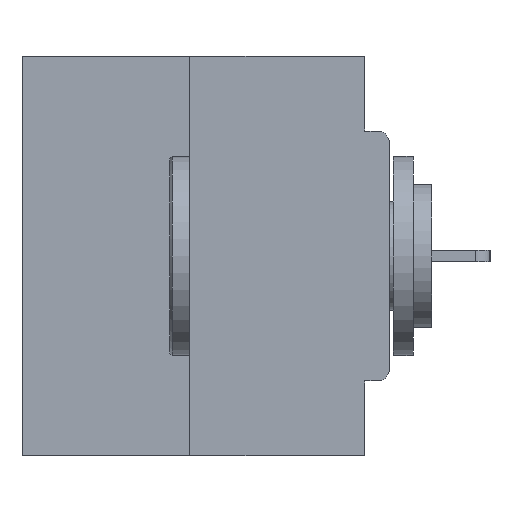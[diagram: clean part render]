
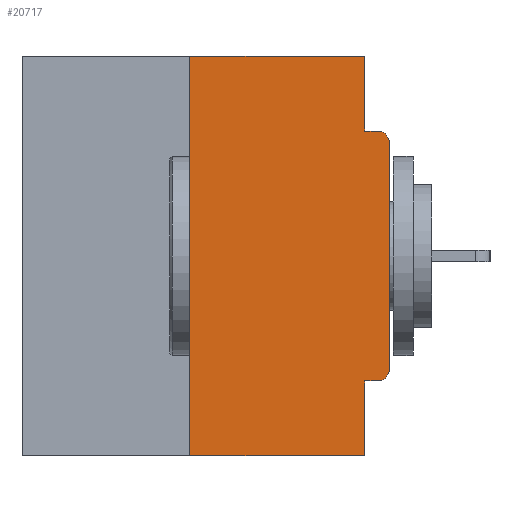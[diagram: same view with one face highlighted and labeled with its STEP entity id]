
A CAD part, left-side view. The second image highlights one B-rep face of the part: STEP entity #20717.
In plain terms, the highlighted planar face has unit normal (-1, 0, 0).
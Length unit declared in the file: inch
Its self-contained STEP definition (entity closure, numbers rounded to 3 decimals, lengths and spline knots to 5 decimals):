
#76 = DIRECTION ( 'NONE',  ( 0., 0., 1. ) ) ;
#214 = VECTOR ( 'NONE', #10319, 39.37008 ) ;
#393 = CARTESIAN_POINT ( 'NONE',  ( 0., 0.46, 0. ) ) ;
#696 = VERTEX_POINT ( 'NONE', #19308 ) ;
#1571 = DIRECTION ( 'NONE',  ( -1., 0., 0. ) ) ;
#2668 = ORIENTED_EDGE ( 'NONE', *, *, #12306, .F. ) ;
#3472 = LINE ( 'NONE', #29844, #12687 ) ;
#3870 = CARTESIAN_POINT ( 'NONE',  ( 0., 0.031, 0. ) ) ;
#4106 = DIRECTION ( 'NONE',  ( 0., 0., -1. ) ) ;
#4189 = PLANE ( 'NONE',  #5320 ) ;
#4296 = DIRECTION ( 'NONE',  ( 0., 0., -1. ) ) ;
#4520 = CARTESIAN_POINT ( 'NONE',  ( 0., 0.015, -0.0935 ) ) ;
#4551 = VERTEX_POINT ( 'NONE', #28477 ) ;
#4788 = VECTOR ( 'NONE', #9952, 39.37008 ) ;
#5167 = VERTEX_POINT ( 'NONE', #29024 ) ;
#5266 = ORIENTED_EDGE ( 'NONE', *, *, #14799, .T. ) ;
#5320 = AXIS2_PLACEMENT_3D ( 'NONE', #6669, #30104, #4296 ) ;
#5883 = EDGE_CURVE ( 'NONE', #19511, #30200, #10725, .T. ) ;
#6249 = VECTOR ( 'NONE', #29331, 39.37008 ) ;
#6626 = ORIENTED_EDGE ( 'NONE', *, *, #5883, .F. ) ;
#6669 = CARTESIAN_POINT ( 'NONE',  ( 0., 0.46, 0. ) ) ;
#6831 = CARTESIAN_POINT ( 'NONE',  ( 0., 0., -0.4065 ) ) ;
#7285 = CARTESIAN_POINT ( 'NONE',  ( 0., 0.031, -0.5 ) ) ;
#8196 = AXIS2_PLACEMENT_3D ( 'NONE', #8327, #22698, #8529 ) ;
#8265 = DIRECTION ( 'NONE',  ( 0., -1., 0. ) ) ;
#8327 = CARTESIAN_POINT ( 'NONE',  ( 0., 0.015, -0.3915 ) ) ;
#8529 = DIRECTION ( 'NONE',  ( 0., 0., -1. ) ) ;
#9159 = VECTOR ( 'NONE', #8265, 39.37008 ) ;
#9408 = CARTESIAN_POINT ( 'NONE',  ( 0., 0.25, 0. ) ) ;
#9952 = DIRECTION ( 'NONE',  ( 0., 0., -1. ) ) ;
#10228 = DIRECTION ( 'NONE',  ( 0., -1., 0. ) ) ;
#10319 = DIRECTION ( 'NONE',  ( 0., 0., 1. ) ) ;
#10347 = CARTESIAN_POINT ( 'NONE',  ( 0., 0.031, -0.4065 ) ) ;
#10432 = CARTESIAN_POINT ( 'NONE',  ( 0., 0., -0.0935 ) ) ;
#10725 = LINE ( 'NONE', #7285, #4788 ) ;
#11297 = VECTOR ( 'NONE', #76, 39.37008 ) ;
#11417 = EDGE_CURVE ( 'NONE', #5167, #19511, #12027, .T. ) ;
#11692 = ORIENTED_EDGE ( 'NONE', *, *, #18692, .T. ) ;
#11786 = ORIENTED_EDGE ( 'NONE', *, *, #16919, .T. ) ;
#12027 = LINE ( 'NONE', #6831, #17896 ) ;
#12306 = EDGE_CURVE ( 'NONE', #4551, #24240, #27589, .T. ) ;
#12375 = CARTESIAN_POINT ( 'NONE',  ( 0., 0., 0. ) ) ;
#12687 = VECTOR ( 'NONE', #15627, 39.37008 ) ;
#12829 = CARTESIAN_POINT ( 'NONE',  ( 0., 0.46, -0.5 ) ) ;
#12853 = VERTEX_POINT ( 'NONE', #9408 ) ;
#12914 = VERTEX_POINT ( 'NONE', #22048 ) ;
#12930 = ORIENTED_EDGE ( 'NONE', *, *, #27582, .F. ) ;
#12961 = AXIS2_PLACEMENT_3D ( 'NONE', #25399, #1571, #4106 ) ;
#13127 = ORIENTED_EDGE ( 'NONE', *, *, #22648, .T. ) ;
#13568 = EDGE_CURVE ( 'NONE', #12914, #12853, #26070, .T. ) ;
#14177 = FACE_OUTER_BOUND ( 'NONE', #26097, .T. ) ;
#14629 = LINE ( 'NONE', #393, #18654 ) ;
#14799 = EDGE_CURVE ( 'NONE', #12914, #30200, #18011, .T. ) ;
#14936 = VERTEX_POINT ( 'NONE', #3870 ) ;
#15118 = ORIENTED_EDGE ( 'NONE', *, *, #13568, .F. ) ;
#15627 = DIRECTION ( 'NONE',  ( 0., 0., -1. ) ) ;
#16919 = EDGE_CURVE ( 'NONE', #5167, #17556, #26741, .T. ) ;
#17556 = VERTEX_POINT ( 'NONE', #20519 ) ;
#17896 = VECTOR ( 'NONE', #28127, 39.37008 ) ;
#18011 = LINE ( 'NONE', #12829, #6249 ) ;
#18089 = CARTESIAN_POINT ( 'NONE',  ( 0., 0.031, -0.5 ) ) ;
#18654 = VECTOR ( 'NONE', #10228, 39.37008 ) ;
#18692 = EDGE_CURVE ( 'NONE', #696, #24240, #27546, .T. ) ;
#19308 = CARTESIAN_POINT ( 'NONE',  ( 0., 0., -0.1085 ) ) ;
#19511 = VERTEX_POINT ( 'NONE', #10347 ) ;
#20519 = CARTESIAN_POINT ( 'NONE',  ( 0., 0., -0.3915 ) ) ;
#20717 = ADVANCED_FACE ( 'NONE', ( #14177 ), #4189, .F. ) ;
#22048 = CARTESIAN_POINT ( 'NONE',  ( 0., 0.25, -0.5 ) ) ;
#22648 = EDGE_CURVE ( 'NONE', #17556, #696, #25656, .T. ) ;
#22698 = DIRECTION ( 'NONE',  ( -1., 0., 0. ) ) ;
#23043 = ORIENTED_EDGE ( 'NONE', *, *, #30102, .F. ) ;
#24240 = VERTEX_POINT ( 'NONE', #4520 ) ;
#25399 = CARTESIAN_POINT ( 'NONE',  ( 0., 0.015, -0.1085 ) ) ;
#25656 = LINE ( 'NONE', #12375, #214 ) ;
#26070 = LINE ( 'NONE', #28343, #11297 ) ;
#26097 = EDGE_LOOP ( 'NONE', ( #12930, #15118, #5266, #6626, #26281, #11786, #13127, #11692, #2668, #23043 ) ) ;
#26281 = ORIENTED_EDGE ( 'NONE', *, *, #11417, .F. ) ;
#26741 = CIRCLE ( 'NONE', #8196, 0.015 ) ;
#27546 = CIRCLE ( 'NONE', #12961, 0.015 ) ;
#27582 = EDGE_CURVE ( 'NONE', #12853, #14936, #14629, .T. ) ;
#27589 = LINE ( 'NONE', #10432, #9159 ) ;
#28127 = DIRECTION ( 'NONE',  ( 0., 1., 0. ) ) ;
#28343 = CARTESIAN_POINT ( 'NONE',  ( 0., 0.25, 0. ) ) ;
#28477 = CARTESIAN_POINT ( 'NONE',  ( 0., 0.031, -0.0935 ) ) ;
#29024 = CARTESIAN_POINT ( 'NONE',  ( 0., 0.015, -0.4065 ) ) ;
#29331 = DIRECTION ( 'NONE',  ( 0., -1., 0. ) ) ;
#29844 = CARTESIAN_POINT ( 'NONE',  ( 0., 0.031, 0. ) ) ;
#30102 = EDGE_CURVE ( 'NONE', #14936, #4551, #3472, .T. ) ;
#30104 = DIRECTION ( 'NONE',  ( 1., 0., 0. ) ) ;
#30200 = VERTEX_POINT ( 'NONE', #18089 ) ;
